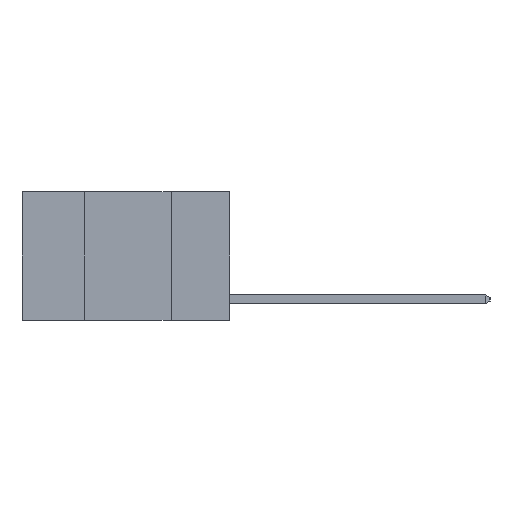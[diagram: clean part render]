
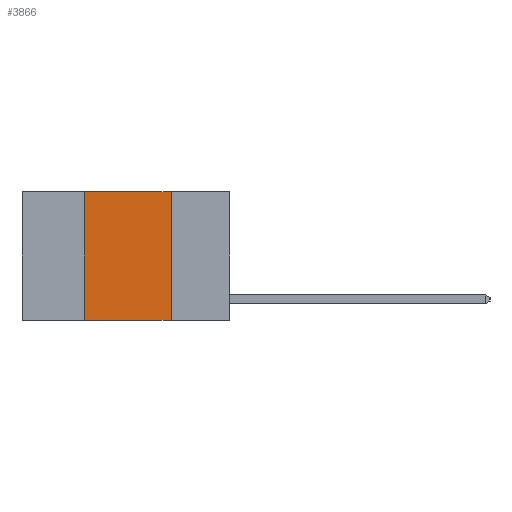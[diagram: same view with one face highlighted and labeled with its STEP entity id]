
A CAD part, left-side view. The second image highlights one B-rep face of the part: STEP entity #3866.
In plain terms, the highlighted planar face has unit normal (-1, 0, 0).
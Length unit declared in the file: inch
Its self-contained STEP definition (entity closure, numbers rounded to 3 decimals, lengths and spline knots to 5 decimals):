
#67 = ORIENTED_EDGE ( 'NONE', *, *, #5560, .F. ) ;
#230 = EDGE_CURVE ( 'NONE', #3626, #6350, #10295, .T. ) ;
#812 = EDGE_CURVE ( 'NONE', #1680, #1128, #6450, .T. ) ;
#1068 = VECTOR ( 'NONE', #3016, 39.37008 ) ;
#1128 = VERTEX_POINT ( 'NONE', #3468 ) ;
#1502 = DIRECTION ( 'NONE',  ( 0., 0., -1. ) ) ;
#1680 = VERTEX_POINT ( 'NONE', #3421 ) ;
#1695 = EDGE_CURVE ( 'NONE', #6350, #1128, #1946, .T. ) ;
#1946 = LINE ( 'NONE', #8163, #7038 ) ;
#2028 = ORIENTED_EDGE ( 'NONE', *, *, #1695, .F. ) ;
#2987 = DIRECTION ( 'NONE',  ( 0., -1., 0. ) ) ;
#3016 = DIRECTION ( 'NONE',  ( 0., -1., 0. ) ) ;
#3421 = CARTESIAN_POINT ( 'NONE',  ( 0., 0.42, -0.37 ) ) ;
#3468 = CARTESIAN_POINT ( 'NONE',  ( 0., 0.17, -0.37 ) ) ;
#3626 = VERTEX_POINT ( 'NONE', #10057 ) ;
#3686 = ORIENTED_EDGE ( 'NONE', *, *, #230, .F. ) ;
#3778 = CARTESIAN_POINT ( 'NONE',  ( 0., 0.42, 0. ) ) ;
#3862 = CARTESIAN_POINT ( 'NONE',  ( 0., 0.6, 0. ) ) ;
#3866 = ADVANCED_FACE ( 'NONE', ( #9732 ), #6639, .F. ) ;
#4776 = DIRECTION ( 'NONE',  ( 0., 0., -1. ) ) ;
#4976 = VECTOR ( 'NONE', #2987, 39.37008 ) ;
#5169 = AXIS2_PLACEMENT_3D ( 'NONE', #7587, #10446, #4776 ) ;
#5560 = EDGE_CURVE ( 'NONE', #1680, #3626, #8650, .T. ) ;
#6350 = VERTEX_POINT ( 'NONE', #10597 ) ;
#6426 = VECTOR ( 'NONE', #11320, 39.37008 ) ;
#6450 = LINE ( 'NONE', #9643, #1068 ) ;
#6639 = PLANE ( 'NONE',  #5169 ) ;
#7038 = VECTOR ( 'NONE', #1502, 39.37008 ) ;
#7587 = CARTESIAN_POINT ( 'NONE',  ( 0., 0.6, 0. ) ) ;
#8163 = CARTESIAN_POINT ( 'NONE',  ( 0., 0.17, 0. ) ) ;
#8650 = LINE ( 'NONE', #3778, #6426 ) ;
#9643 = CARTESIAN_POINT ( 'NONE',  ( 0., 0.6, -0.37 ) ) ;
#9732 = FACE_OUTER_BOUND ( 'NONE', #10468, .T. ) ;
#9909 = ORIENTED_EDGE ( 'NONE', *, *, #812, .T. ) ;
#10057 = CARTESIAN_POINT ( 'NONE',  ( 0., 0.42, 0. ) ) ;
#10295 = LINE ( 'NONE', #3862, #4976 ) ;
#10446 = DIRECTION ( 'NONE',  ( 1., 0., 0. ) ) ;
#10468 = EDGE_LOOP ( 'NONE', ( #2028, #3686, #67, #9909 ) ) ;
#10597 = CARTESIAN_POINT ( 'NONE',  ( 0., 0.17, 0. ) ) ;
#11320 = DIRECTION ( 'NONE',  ( 0., 0., 1. ) ) ;
